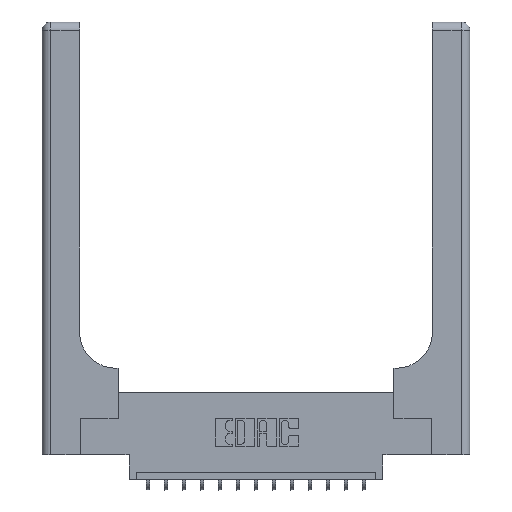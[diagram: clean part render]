
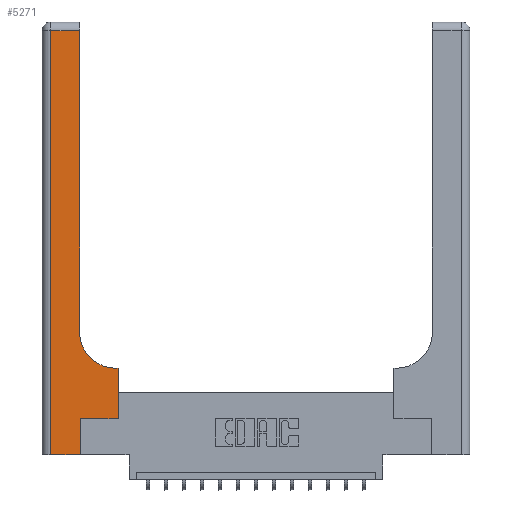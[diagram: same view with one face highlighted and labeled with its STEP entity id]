
A CAD part, top view. The second image highlights one B-rep face of the part: STEP entity #5271.
In plain terms, the highlighted planar face has unit normal (0, 0, 1).
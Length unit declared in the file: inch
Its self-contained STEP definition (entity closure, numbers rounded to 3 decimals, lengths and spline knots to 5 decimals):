
#77 = CARTESIAN_POINT ( 'NONE',  ( 0.528, 0.6, 0.37 ) ) ;
#279 = LINE ( 'NONE', #4621, #11609 ) ;
#308 = CARTESIAN_POINT ( 'NONE',  ( 0.26, 2.94, 0.37 ) ) ;
#339 = VECTOR ( 'NONE', #6864, 39.37008 ) ;
#886 = ORIENTED_EDGE ( 'NONE', *, *, #1136, .T. ) ;
#1064 = ORIENTED_EDGE ( 'NONE', *, *, #4240, .T. ) ;
#1136 = EDGE_CURVE ( 'NONE', #3430, #4804, #9551, .T. ) ;
#1176 = VERTEX_POINT ( 'NONE', #308 ) ;
#1456 = DIRECTION ( 'NONE',  ( -1., 0., 0. ) ) ;
#1467 = CARTESIAN_POINT ( 'NONE',  ( 0.26, 0.6, 0.37 ) ) ;
#1490 = LINE ( 'NONE', #4563, #17675 ) ;
#1825 = DIRECTION ( 'NONE',  ( 0., -1., 0. ) ) ;
#1855 = DIRECTION ( 'NONE',  ( 0., 0., -1. ) ) ;
#1889 = EDGE_CURVE ( 'NONE', #1176, #4089, #5017, .T. ) ;
#2128 = CARTESIAN_POINT ( 'NONE',  ( 0.06, 2.94, 0.37 ) ) ;
#2858 = EDGE_CURVE ( 'NONE', #17567, #15779, #6368, .T. ) ;
#3053 = DIRECTION ( 'NONE',  ( 0., 1., 0. ) ) ;
#3430 = VERTEX_POINT ( 'NONE', #17679 ) ;
#4089 = VERTEX_POINT ( 'NONE', #2128 ) ;
#4149 = PLANE ( 'NONE',  #11074 ) ;
#4240 = EDGE_CURVE ( 'NONE', #4089, #9852, #279, .T. ) ;
#4390 = EDGE_CURVE ( 'NONE', #9852, #10561, #16206, .T. ) ;
#4563 = CARTESIAN_POINT ( 'NONE',  ( 0.528, 0.25, 0.37 ) ) ;
#4621 = CARTESIAN_POINT ( 'NONE',  ( 0.06, 3., 0.37 ) ) ;
#4804 = VERTEX_POINT ( 'NONE', #9174 ) ;
#5017 = LINE ( 'NONE', #9280, #12126 ) ;
#5271 = ADVANCED_FACE ( 'NONE', ( #5431 ), #4149, .F. ) ;
#5431 = FACE_OUTER_BOUND ( 'NONE', #8263, .T. ) ;
#5521 = LINE ( 'NONE', #16727, #13610 ) ;
#5743 = CARTESIAN_POINT ( 'NONE',  ( 0.51, 0.6, 0.37 ) ) ;
#5999 = CARTESIAN_POINT ( 'NONE',  ( 0.51, 0.85, 0.37 ) ) ;
#6368 = CIRCLE ( 'NONE', #14685, 0.25 ) ;
#6763 = CARTESIAN_POINT ( 'NONE',  ( 0.26, 0.85, 0.37 ) ) ;
#6864 = DIRECTION ( 'NONE',  ( 1., 0., 0. ) ) ;
#7140 = ORIENTED_EDGE ( 'NONE', *, *, #1889, .T. ) ;
#7204 = ORIENTED_EDGE ( 'NONE', *, *, #8759, .T. ) ;
#7594 = DIRECTION ( 'NONE',  ( -1., 0., 0. ) ) ;
#8263 = EDGE_LOOP ( 'NONE', ( #7204, #7140, #1064, #11646, #9450, #886, #14770, #11513, #17510 ) ) ;
#8759 = EDGE_CURVE ( 'NONE', #15779, #1176, #5521, .T. ) ;
#8988 = EDGE_CURVE ( 'NONE', #4804, #10239, #1490, .T. ) ;
#9046 = CARTESIAN_POINT ( 'NONE',  ( 0.265, 0., 0.37 ) ) ;
#9167 = CARTESIAN_POINT ( 'NONE',  ( 0., 0., 0.37 ) ) ;
#9174 = CARTESIAN_POINT ( 'NONE',  ( 0.528, 0.25, 0.37 ) ) ;
#9280 = CARTESIAN_POINT ( 'NONE',  ( 0., 2.94, 0.37 ) ) ;
#9421 = DIRECTION ( 'NONE',  ( 0., 1., 0. ) ) ;
#9450 = ORIENTED_EDGE ( 'NONE', *, *, #15043, .T. ) ;
#9551 = LINE ( 'NONE', #13682, #339 ) ;
#9852 = VERTEX_POINT ( 'NONE', #11269 ) ;
#10239 = VERTEX_POINT ( 'NONE', #77 ) ;
#10561 = VERTEX_POINT ( 'NONE', #9046 ) ;
#10917 = VECTOR ( 'NONE', #13495, 39.37008 ) ;
#11074 = AXIS2_PLACEMENT_3D ( 'NONE', #12168, #15119, #1456 ) ;
#11269 = CARTESIAN_POINT ( 'NONE',  ( 0.06, 0., 0.37 ) ) ;
#11513 = ORIENTED_EDGE ( 'NONE', *, *, #14657, .T. ) ;
#11609 = VECTOR ( 'NONE', #1825, 39.37008 ) ;
#11646 = ORIENTED_EDGE ( 'NONE', *, *, #4390, .T. ) ;
#12126 = VECTOR ( 'NONE', #7594, 39.37008 ) ;
#12168 = CARTESIAN_POINT ( 'NONE',  ( 0., 3., 0.37 ) ) ;
#12318 = CARTESIAN_POINT ( 'NONE',  ( 0.265, 0., 0.37 ) ) ;
#13315 = DIRECTION ( 'NONE',  ( 1., 0., 0. ) ) ;
#13495 = DIRECTION ( 'NONE',  ( -1., 0., 0. ) ) ;
#13610 = VECTOR ( 'NONE', #3053, 39.37008 ) ;
#13682 = CARTESIAN_POINT ( 'NONE',  ( 0.265, 0.25, 0.37 ) ) ;
#13747 = LINE ( 'NONE', #1467, #10917 ) ;
#13750 = VECTOR ( 'NONE', #9421, 39.37008 ) ;
#14657 = EDGE_CURVE ( 'NONE', #10239, #17567, #13747, .T. ) ;
#14685 = AXIS2_PLACEMENT_3D ( 'NONE', #5999, #1855, #15352 ) ;
#14770 = ORIENTED_EDGE ( 'NONE', *, *, #8988, .T. ) ;
#15043 = EDGE_CURVE ( 'NONE', #10561, #3430, #15113, .T. ) ;
#15113 = LINE ( 'NONE', #12318, #13750 ) ;
#15119 = DIRECTION ( 'NONE',  ( 0., 0., -1. ) ) ;
#15352 = DIRECTION ( 'NONE',  ( 1., 0., 0. ) ) ;
#15779 = VERTEX_POINT ( 'NONE', #6763 ) ;
#16206 = LINE ( 'NONE', #9167, #17055 ) ;
#16727 = CARTESIAN_POINT ( 'NONE',  ( 0.26, 3., 0.37 ) ) ;
#16961 = DIRECTION ( 'NONE',  ( 0., 1., 0. ) ) ;
#17055 = VECTOR ( 'NONE', #13315, 39.37008 ) ;
#17510 = ORIENTED_EDGE ( 'NONE', *, *, #2858, .T. ) ;
#17567 = VERTEX_POINT ( 'NONE', #5743 ) ;
#17675 = VECTOR ( 'NONE', #16961, 39.37008 ) ;
#17679 = CARTESIAN_POINT ( 'NONE',  ( 0.265, 0.25, 0.37 ) ) ;
